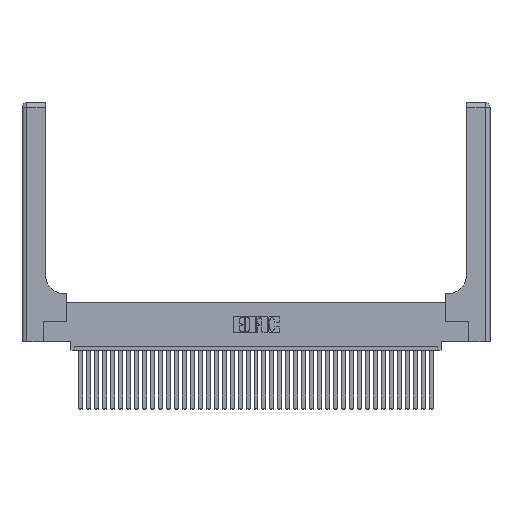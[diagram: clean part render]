
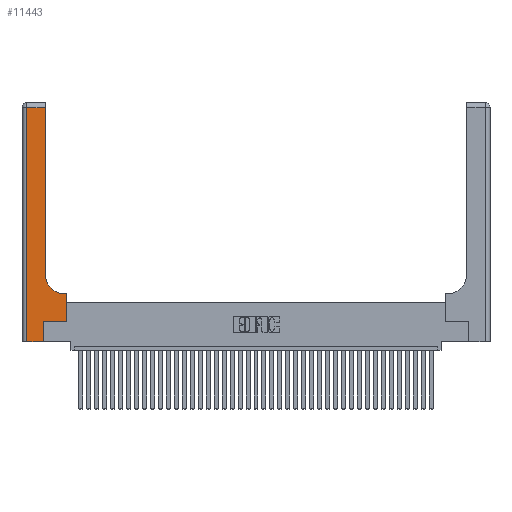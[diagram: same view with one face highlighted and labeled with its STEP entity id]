
A CAD part, top view. The second image highlights one B-rep face of the part: STEP entity #11443.
In plain terms, the highlighted planar face has unit normal (0, 0, 1).
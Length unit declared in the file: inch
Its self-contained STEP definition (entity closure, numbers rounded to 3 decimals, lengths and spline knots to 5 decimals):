
#271 = EDGE_CURVE ( 'NONE', #32146, #27082, #38080, .T. ) ;
#1287 = CARTESIAN_POINT ( 'NONE',  ( 0., 3., 0.37 ) ) ;
#1400 = LINE ( 'NONE', #10148, #7020 ) ;
#1673 = VERTEX_POINT ( 'NONE', #35246 ) ;
#1711 = EDGE_LOOP ( 'NONE', ( #34454, #2573, #6899, #31218, #8449, #28264, #8992, #32065, #2960 ) ) ;
#1739 = VERTEX_POINT ( 'NONE', #13883 ) ;
#2179 = CARTESIAN_POINT ( 'NONE',  ( 0.2915, 0.6, 0.37 ) ) ;
#2573 = ORIENTED_EDGE ( 'NONE', *, *, #22409, .T. ) ;
#2960 = ORIENTED_EDGE ( 'NONE', *, *, #18240, .T. ) ;
#4193 = VERTEX_POINT ( 'NONE', #6824 ) ;
#5490 = VECTOR ( 'NONE', #37713, 39.37008 ) ;
#6021 = EDGE_CURVE ( 'NONE', #27082, #27279, #35031, .T. ) ;
#6546 = VECTOR ( 'NONE', #27585, 39.37008 ) ;
#6713 = DIRECTION ( 'NONE',  ( -1., 0., 0. ) ) ;
#6824 = CARTESIAN_POINT ( 'NONE',  ( 0.2915, 2.94, 0.37 ) ) ;
#6871 = LINE ( 'NONE', #2179, #5490 ) ;
#6899 = ORIENTED_EDGE ( 'NONE', *, *, #271, .T. ) ;
#7020 = VECTOR ( 'NONE', #31416, 39.37008 ) ;
#7035 = EDGE_CURVE ( 'NONE', #1673, #31866, #9688, .T. ) ;
#7614 = CARTESIAN_POINT ( 'NONE',  ( 0.2915, 3., 0.37 ) ) ;
#7824 = DIRECTION ( 'NONE',  ( 0., -1., 0. ) ) ;
#8449 = ORIENTED_EDGE ( 'NONE', *, *, #26404, .T. ) ;
#8992 = ORIENTED_EDGE ( 'NONE', *, *, #28645, .T. ) ;
#9688 = LINE ( 'NONE', #9995, #25517 ) ;
#9995 = CARTESIAN_POINT ( 'NONE',  ( 0.269, 0.25, 0.37 ) ) ;
#10148 = CARTESIAN_POINT ( 'NONE',  ( 0.269, 0., 0.37 ) ) ;
#10799 = VERTEX_POINT ( 'NONE', #36922 ) ;
#11443 = ADVANCED_FACE ( 'NONE', ( #12933 ), #19149, .F. ) ;
#12755 = EDGE_CURVE ( 'NONE', #1739, #4193, #26885, .T. ) ;
#12933 = FACE_OUTER_BOUND ( 'NONE', #1711, .T. ) ;
#13883 = CARTESIAN_POINT ( 'NONE',  ( 0.2915, 0.85, 0.37 ) ) ;
#16005 = DIRECTION ( 'NONE',  ( 0., 1., 0. ) ) ;
#16878 = VERTEX_POINT ( 'NONE', #26816 ) ;
#18240 = EDGE_CURVE ( 'NONE', #10799, #1739, #38138, .T. ) ;
#19149 = PLANE ( 'NONE',  #35878 ) ;
#19217 = CARTESIAN_POINT ( 'NONE',  ( 0.5585, 0.25, 0.37 ) ) ;
#21569 = VECTOR ( 'NONE', #16005, 39.37008 ) ;
#21711 = AXIS2_PLACEMENT_3D ( 'NONE', #27739, #36320, #36689 ) ;
#22106 = DIRECTION ( 'NONE',  ( -1., 0., 0. ) ) ;
#22409 = EDGE_CURVE ( 'NONE', #4193, #32146, #33635, .T. ) ;
#22524 = LINE ( 'NONE', #19217, #21569 ) ;
#23339 = CARTESIAN_POINT ( 'NONE',  ( 0.5585, 0.25, 0.37 ) ) ;
#24654 = EDGE_CURVE ( 'NONE', #16878, #10799, #6871, .T. ) ;
#24999 = CARTESIAN_POINT ( 'NONE',  ( 0.06, 3., 0.37 ) ) ;
#25517 = VECTOR ( 'NONE', #33821, 39.37008 ) ;
#25545 = CARTESIAN_POINT ( 'NONE',  ( 0.06, 2.94, 0.37 ) ) ;
#25977 = CARTESIAN_POINT ( 'NONE',  ( 0.06, 0., 0.37 ) ) ;
#26404 = EDGE_CURVE ( 'NONE', #27279, #1673, #1400, .T. ) ;
#26816 = CARTESIAN_POINT ( 'NONE',  ( 0.5585, 0.6, 0.37 ) ) ;
#26885 = LINE ( 'NONE', #7614, #29736 ) ;
#27082 = VERTEX_POINT ( 'NONE', #25977 ) ;
#27279 = VERTEX_POINT ( 'NONE', #29286 ) ;
#27585 = DIRECTION ( 'NONE',  ( 1., 0., 0. ) ) ;
#27739 = CARTESIAN_POINT ( 'NONE',  ( 0.5415, 0.85, 0.37 ) ) ;
#27905 = DIRECTION ( 'NONE',  ( 0., 0., -1. ) ) ;
#28264 = ORIENTED_EDGE ( 'NONE', *, *, #7035, .T. ) ;
#28645 = EDGE_CURVE ( 'NONE', #31866, #16878, #22524, .T. ) ;
#29024 = VECTOR ( 'NONE', #6713, 39.37008 ) ;
#29286 = CARTESIAN_POINT ( 'NONE',  ( 0.269, 0., 0.37 ) ) ;
#29736 = VECTOR ( 'NONE', #34451, 39.37008 ) ;
#30210 = CARTESIAN_POINT ( 'NONE',  ( 0., 2.94, 0.37 ) ) ;
#31218 = ORIENTED_EDGE ( 'NONE', *, *, #6021, .T. ) ;
#31416 = DIRECTION ( 'NONE',  ( 0., 1., 0. ) ) ;
#31866 = VERTEX_POINT ( 'NONE', #23339 ) ;
#32065 = ORIENTED_EDGE ( 'NONE', *, *, #24654, .T. ) ;
#32146 = VERTEX_POINT ( 'NONE', #25545 ) ;
#33635 = LINE ( 'NONE', #30210, #29024 ) ;
#33821 = DIRECTION ( 'NONE',  ( 1., 0., 0. ) ) ;
#34364 = VECTOR ( 'NONE', #7824, 39.37008 ) ;
#34451 = DIRECTION ( 'NONE',  ( 0., 1., 0. ) ) ;
#34454 = ORIENTED_EDGE ( 'NONE', *, *, #12755, .T. ) ;
#35031 = LINE ( 'NONE', #36666, #6546 ) ;
#35246 = CARTESIAN_POINT ( 'NONE',  ( 0.269, 0.25, 0.37 ) ) ;
#35878 = AXIS2_PLACEMENT_3D ( 'NONE', #1287, #27905, #22106 ) ;
#36320 = DIRECTION ( 'NONE',  ( 0., 0., -1. ) ) ;
#36666 = CARTESIAN_POINT ( 'NONE',  ( 0., 0., 0.37 ) ) ;
#36689 = DIRECTION ( 'NONE',  ( 1., 0., 0. ) ) ;
#36922 = CARTESIAN_POINT ( 'NONE',  ( 0.5415, 0.6, 0.37 ) ) ;
#37713 = DIRECTION ( 'NONE',  ( -1., 0., 0. ) ) ;
#38080 = LINE ( 'NONE', #24999, #34364 ) ;
#38138 = CIRCLE ( 'NONE', #21711, 0.25 ) ;
